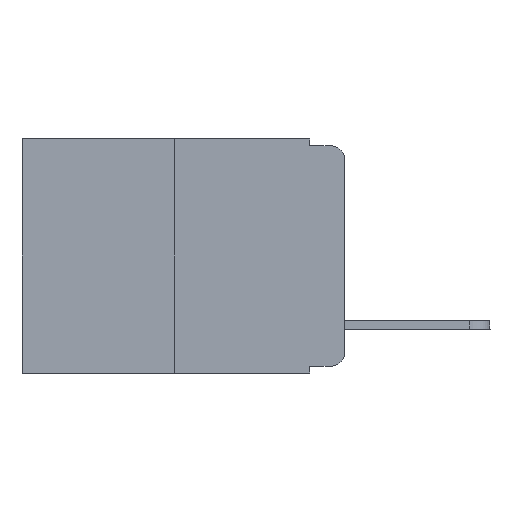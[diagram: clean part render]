
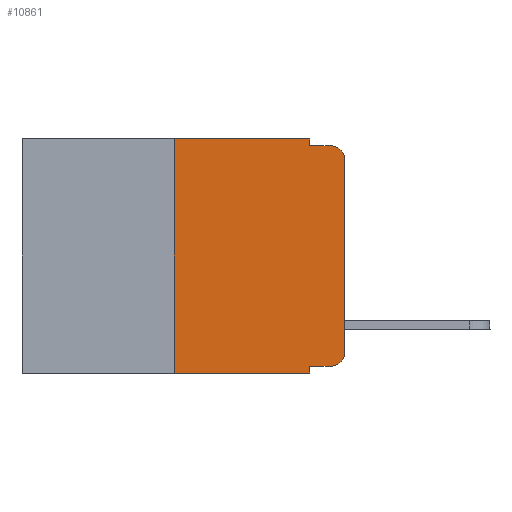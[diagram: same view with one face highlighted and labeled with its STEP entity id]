
A CAD part, left-side view. The second image highlights one B-rep face of the part: STEP entity #10861.
In plain terms, the highlighted planar face has unit normal (-1, 0, 0).
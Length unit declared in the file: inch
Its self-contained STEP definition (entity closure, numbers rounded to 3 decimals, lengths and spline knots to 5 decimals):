
#510 = CARTESIAN_POINT ( 'NONE',  ( 0., 0.02, -0.01 ) ) ;
#699 = DIRECTION ( 'NONE',  ( 1., 0., 0. ) ) ;
#772 = VECTOR ( 'NONE', #9540, 39.37008 ) ;
#784 = CARTESIAN_POINT ( 'NONE',  ( 0., 0.25, 0. ) ) ;
#1642 = DIRECTION ( 'NONE',  ( 0., -1., 0. ) ) ;
#1714 = VECTOR ( 'NONE', #3883, 39.37008 ) ;
#2003 = ORIENTED_EDGE ( 'NONE', *, *, #7081, .F. ) ;
#2475 = DIRECTION ( 'NONE',  ( 0., 0., -1. ) ) ;
#2566 = VECTOR ( 'NONE', #10954, 39.37008 ) ;
#2829 = CARTESIAN_POINT ( 'NONE',  ( 0., 0.02, -0.333 ) ) ;
#3279 = VECTOR ( 'NONE', #19368, 39.37008 ) ;
#3664 = EDGE_CURVE ( 'NONE', #15512, #10672, #15083, .T. ) ;
#3883 = DIRECTION ( 'NONE',  ( 0., -1., 0. ) ) ;
#4133 = EDGE_LOOP ( 'NONE', ( #10692, #10838, #18520, #17401, #13674, #13281, #15674, #2003, #15556, #12714 ) ) ;
#4408 = CARTESIAN_POINT ( 'NONE',  ( 0., 0.051, 0. ) ) ;
#4476 = VERTEX_POINT ( 'NONE', #6171 ) ;
#4825 = LINE ( 'NONE', #4927, #2566 ) ;
#4927 = CARTESIAN_POINT ( 'NONE',  ( 0., 0.051, 0. ) ) ;
#5101 = EDGE_CURVE ( 'NONE', #13126, #6534, #12840, .T. ) ;
#5127 = DIRECTION ( 'NONE',  ( 0., 0., -1. ) ) ;
#5385 = CARTESIAN_POINT ( 'NONE',  ( 0., 0.473, -0.343 ) ) ;
#5512 = LINE ( 'NONE', #8668, #9201 ) ;
#5517 = AXIS2_PLACEMENT_3D ( 'NONE', #6622, #18830, #8102 ) ;
#6171 = CARTESIAN_POINT ( 'NONE',  ( 0., 0.051, -0.343 ) ) ;
#6222 = CARTESIAN_POINT ( 'NONE',  ( 0., 0.051, -0.01 ) ) ;
#6534 = VERTEX_POINT ( 'NONE', #6222 ) ;
#6622 = CARTESIAN_POINT ( 'NONE',  ( 0., 0.02, -0.03 ) ) ;
#6812 = DIRECTION ( 'NONE',  ( 0., 0., 1. ) ) ;
#7081 = EDGE_CURVE ( 'NONE', #7130, #4476, #4825, .T. ) ;
#7130 = VERTEX_POINT ( 'NONE', #18609 ) ;
#7626 = CARTESIAN_POINT ( 'NONE',  ( 0., 0., -0.313 ) ) ;
#7883 = VECTOR ( 'NONE', #2475, 39.37008 ) ;
#8047 = VECTOR ( 'NONE', #6812, 39.37008 ) ;
#8077 = CARTESIAN_POINT ( 'NONE',  ( 0., 0.25, 0. ) ) ;
#8102 = DIRECTION ( 'NONE',  ( 0., 0., -1. ) ) ;
#8112 = DIRECTION ( 'NONE',  ( 0., 0., -1. ) ) ;
#8668 = CARTESIAN_POINT ( 'NONE',  ( 0., 0.051, -0.333 ) ) ;
#8842 = AXIS2_PLACEMENT_3D ( 'NONE', #15659, #699, #8112 ) ;
#8914 = EDGE_CURVE ( 'NONE', #12881, #4476, #12883, .T. ) ;
#9201 = VECTOR ( 'NONE', #12725, 39.37008 ) ;
#9540 = DIRECTION ( 'NONE',  ( 0., 0., 1. ) ) ;
#9602 = PLANE ( 'NONE',  #8842 ) ;
#10502 = CARTESIAN_POINT ( 'NONE',  ( 0., 0.473, 0. ) ) ;
#10672 = VERTEX_POINT ( 'NONE', #7626 ) ;
#10692 = ORIENTED_EDGE ( 'NONE', *, *, #14366, .T. ) ;
#10727 = LINE ( 'NONE', #18391, #13661 ) ;
#10838 = ORIENTED_EDGE ( 'NONE', *, *, #15360, .T. ) ;
#10861 = ADVANCED_FACE ( 'NONE', ( #14068 ), #9602, .F. ) ;
#10954 = DIRECTION ( 'NONE',  ( 0., 0., -1. ) ) ;
#10967 = AXIS2_PLACEMENT_3D ( 'NONE', #12544, #11250, #5127 ) ;
#11250 = DIRECTION ( 'NONE',  ( -1., 0., 0. ) ) ;
#11415 = EDGE_CURVE ( 'NONE', #6534, #12378, #10727, .T. ) ;
#12212 = LINE ( 'NONE', #15302, #772 ) ;
#12378 = VERTEX_POINT ( 'NONE', #510 ) ;
#12508 = EDGE_CURVE ( 'NONE', #7130, #15512, #5512, .T. ) ;
#12544 = CARTESIAN_POINT ( 'NONE',  ( 0., 0.02, -0.313 ) ) ;
#12714 = ORIENTED_EDGE ( 'NONE', *, *, #3664, .T. ) ;
#12725 = DIRECTION ( 'NONE',  ( 0., -1., 0. ) ) ;
#12840 = LINE ( 'NONE', #12940, #7883 ) ;
#12881 = VERTEX_POINT ( 'NONE', #16093 ) ;
#12883 = LINE ( 'NONE', #5385, #1714 ) ;
#12940 = CARTESIAN_POINT ( 'NONE',  ( 0., 0.051, 0. ) ) ;
#13092 = CIRCLE ( 'NONE', #5517, 0.02 ) ;
#13126 = VERTEX_POINT ( 'NONE', #4408 ) ;
#13281 = ORIENTED_EDGE ( 'NONE', *, *, #15393, .F. ) ;
#13498 = EDGE_CURVE ( 'NONE', #19441, #13126, #19464, .T. ) ;
#13661 = VECTOR ( 'NONE', #1642, 39.37008 ) ;
#13674 = ORIENTED_EDGE ( 'NONE', *, *, #13498, .F. ) ;
#14068 = FACE_OUTER_BOUND ( 'NONE', #4133, .T. ) ;
#14366 = EDGE_CURVE ( 'NONE', #10672, #17192, #12212, .T. ) ;
#15083 = CIRCLE ( 'NONE', #10967, 0.02 ) ;
#15302 = CARTESIAN_POINT ( 'NONE',  ( 0., 0., 0. ) ) ;
#15360 = EDGE_CURVE ( 'NONE', #17192, #12378, #13092, .T. ) ;
#15393 = EDGE_CURVE ( 'NONE', #12881, #19441, #15742, .T. ) ;
#15512 = VERTEX_POINT ( 'NONE', #2829 ) ;
#15556 = ORIENTED_EDGE ( 'NONE', *, *, #12508, .T. ) ;
#15659 = CARTESIAN_POINT ( 'NONE',  ( 0., 0.473, 0. ) ) ;
#15674 = ORIENTED_EDGE ( 'NONE', *, *, #8914, .T. ) ;
#15742 = LINE ( 'NONE', #784, #8047 ) ;
#16093 = CARTESIAN_POINT ( 'NONE',  ( 0., 0.25, -0.343 ) ) ;
#16870 = CARTESIAN_POINT ( 'NONE',  ( 0., 0., -0.03 ) ) ;
#17192 = VERTEX_POINT ( 'NONE', #16870 ) ;
#17401 = ORIENTED_EDGE ( 'NONE', *, *, #5101, .F. ) ;
#18391 = CARTESIAN_POINT ( 'NONE',  ( 0., 0.051, -0.01 ) ) ;
#18520 = ORIENTED_EDGE ( 'NONE', *, *, #11415, .F. ) ;
#18609 = CARTESIAN_POINT ( 'NONE',  ( 0., 0.051, -0.333 ) ) ;
#18830 = DIRECTION ( 'NONE',  ( -1., 0., 0. ) ) ;
#19368 = DIRECTION ( 'NONE',  ( 0., -1., 0. ) ) ;
#19441 = VERTEX_POINT ( 'NONE', #8077 ) ;
#19464 = LINE ( 'NONE', #10502, #3279 ) ;
